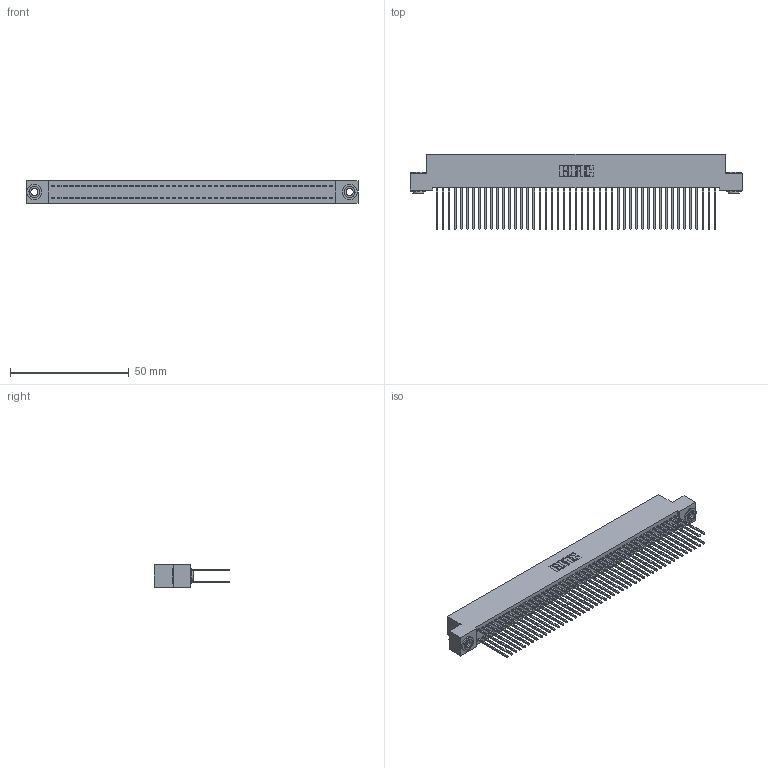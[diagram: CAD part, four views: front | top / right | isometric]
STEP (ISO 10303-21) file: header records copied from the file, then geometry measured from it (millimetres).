
FILE_DESCRIPTION (( 'STEP AP203' ), '1' );
FILE_NAME ('342-094-542-203.STEP', '2018-08-14T02:33:29', ( '' ), ( '' ), 'SwSTEP 2.0', 'SolidWorks 2016', '' );
FILE_SCHEMA (( 'CONFIG_CONTROL_DESIGN' ));
Length unit declared in the file: inch
Products named in the file (4): 342 Part_.156 TH; 345-292-001_345-293-142; 342-250-002_345-250-002-102; 342-094-542-203
Assembly tree (97 placements, depth 2):
  342-094-542-203
    342 Part_.156 TH
    345-292-001_345-293-142  x94
    342-250-002_345-250-002-102  x2
Bounding box: 139.7 x 31.63 x 9.4 mm (x, y, z)
Volume: 13036.7 mm3; surface area: 23524.2 mm2
Topology: 97 solids, 97 shells, 5036 faces, 14945 edges, 9834 vertices
Faces by surface type: plane 3460, cylinder 1568, cone 8
Entity records: 30126 total; most frequent: CARTESIAN_POINT 4961, ORIENTED_EDGE 4890, DIRECTION 4263, EDGE_CURVE 2445, LINE 2293, VECTOR 2293, VERTEX_POINT 1626, AXIS2_PLACEMENT_3D 985
